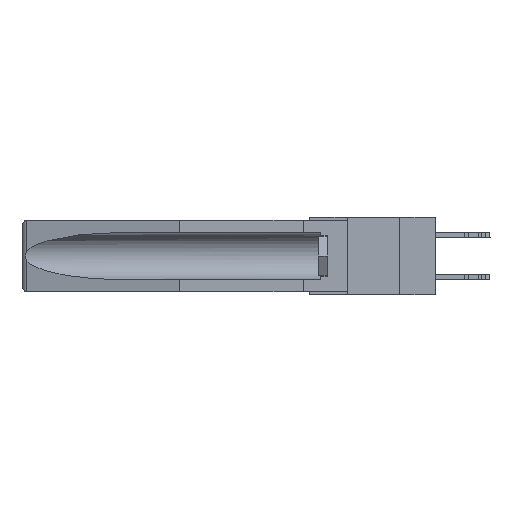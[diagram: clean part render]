
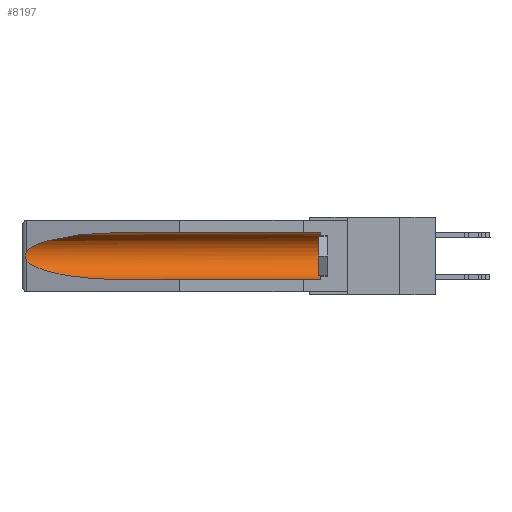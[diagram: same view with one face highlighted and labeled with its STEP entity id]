
A CAD part, left-side view. The second image highlights one B-rep face of the part: STEP entity #8197.
In plain terms, the highlighted cylindrical face has radius 2.857 mm (diameter 5.715 mm), a partial arc.
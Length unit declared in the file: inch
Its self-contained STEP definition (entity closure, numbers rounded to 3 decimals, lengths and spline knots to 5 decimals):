
#488 = CARTESIAN_POINT ( 'NONE',  ( 0.21114, 1.30732, -0.284 ) ) ;
#608 = CARTESIAN_POINT ( 'NONE',  ( 0.25451, 1.48313, -0.24835 ) ) ;
#1193 = CARTESIAN_POINT ( 'NONE',  ( 0.26537, 1.52718, -0.14972 ) ) ;
#1194 = CARTESIAN_POINT ( 'NONE',  ( 0.26537, 1.52718, -0.19328 ) ) ;
#2556 = DIRECTION ( 'NONE',  ( 0., 1., 0. ) ) ;
#3666 = VERTEX_POINT ( 'NONE', #18218 ) ;
#4886 = FACE_OUTER_BOUND ( 'NONE', #32067, .T. ) ;
#5079 = CARTESIAN_POINT ( 'NONE',  ( 0.26537, 1.52718, -0.14972 ) ) ;
#5500 = LINE ( 'NONE', #27120, #18323 ) ;
#5696 = EDGE_CURVE ( 'NONE', #31423, #12326, #31787, .T. ) ;
#6207 = ORIENTED_EDGE ( 'NONE', *, *, #6309, .F. ) ;
#6309 = EDGE_CURVE ( 'NONE', #16053, #23123, #12620, .T. ) ;
#6345 = ORIENTED_EDGE ( 'NONE', *, *, #5696, .T. ) ;
#7160 = CARTESIAN_POINT ( 'NONE',  ( 0.2673, 1.5327, -0.16383 ) ) ;
#7705 = CARTESIAN_POINT ( 'NONE',  ( 0.155, 1.07973, -0.284 ) ) ;
#8197 = ADVANCED_FACE ( 'NONE', ( #4886 ), #17711, .F. ) ;
#8872 = ORIENTED_EDGE ( 'NONE', *, *, #15771, .T. ) ;
#9637 = CARTESIAN_POINT ( 'NONE',  ( 0.26654, 1.53092, -0.15636 ) ) ;
#9998 = DIRECTION ( 'NONE',  ( 0., 0., 1. ) ) ;
#10888 =( BOUNDED_CURVE ( )  B_SPLINE_CURVE ( 3, ( #10934, #608, #488, #23588 ),
 .UNSPECIFIED., .F., .F. ) 
 B_SPLINE_CURVE_WITH_KNOTS ( ( 4, 4 ),
 ( 0.1948, 1.5708 ),
 .UNSPECIFIED. ) 
 CURVE ( )  GEOMETRIC_REPRESENTATION_ITEM ( )  RATIONAL_B_SPLINE_CURVE ( ( 1., 0.848, 0.848, 1. ) ) 
 REPRESENTATION_ITEM ( '' )  );
#10934 = CARTESIAN_POINT ( 'NONE',  ( 0.26537, 1.52718, -0.19328 ) ) ;
#11976 = EDGE_CURVE ( 'NONE', #16053, #21018, #19033, .T. ) ;
#12223 = CARTESIAN_POINT ( 'NONE',  ( 0.155, -0.30754, -0.284 ) ) ;
#12326 = VERTEX_POINT ( 'NONE', #1193 ) ;
#12581 = ORIENTED_EDGE ( 'NONE', *, *, #17469, .T. ) ;
#12620 = LINE ( 'NONE', #12223, #29821 ) ;
#13953 = CARTESIAN_POINT ( 'NONE',  ( 0.26655, 1.53094, -0.18657 ) ) ;
#14879 = CARTESIAN_POINT ( 'NONE',  ( 0.155, 1.07973, -0.059 ) ) ;
#15127 = ORIENTED_EDGE ( 'NONE', *, *, #11976, .T. ) ;
#15260 = DIRECTION ( 'NONE',  ( 0., 1., 0. ) ) ;
#15278 = CARTESIAN_POINT ( 'NONE',  ( 0.25451, 1.48313, -0.09465 ) ) ;
#15771 = EDGE_CURVE ( 'NONE', #12326, #3666, #16846, .T. ) ;
#16053 = VERTEX_POINT ( 'NONE', #25315 ) ;
#16846 = B_SPLINE_CURVE_WITH_KNOTS ( 'NONE', 3,
 ( #27351, #22171, #9637, #7160, #26981, #29516, #27090, #13953, #32079, #1194 ),
 .UNSPECIFIED., .F., .F.,
 ( 4, 2, 2, 2, 4 ),
 ( 0., 0.00029, 0.00058, 0.00087, 0.00117 ),
 .UNSPECIFIED. ) ;
#17469 = EDGE_CURVE ( 'NONE', #3666, #23123, #10888, .T. ) ;
#17711 = CYLINDRICAL_SURFACE ( 'NONE', #21744, 0.1125 ) ;
#18218 = CARTESIAN_POINT ( 'NONE',  ( 0.26537, 1.52718, -0.19328 ) ) ;
#18323 = VECTOR ( 'NONE', #33009, 39.37008 ) ;
#18968 = EDGE_CURVE ( 'NONE', #21018, #31423, #5500, .T. ) ;
#19033 = CIRCLE ( 'NONE', #23303, 0.1125 ) ;
#19790 = DIRECTION ( 'NONE',  ( 0., -1., 0. ) ) ;
#20298 = CARTESIAN_POINT ( 'NONE',  ( 0.155, 1.07973, -0.059 ) ) ;
#21018 = VERTEX_POINT ( 'NONE', #28309 ) ;
#21744 = AXIS2_PLACEMENT_3D ( 'NONE', #25343, #15260, #9998 ) ;
#22171 = CARTESIAN_POINT ( 'NONE',  ( 0.26597, 1.52961, -0.15275 ) ) ;
#22893 = CARTESIAN_POINT ( 'NONE',  ( 0.21114, 1.30732, -0.059 ) ) ;
#23123 = VERTEX_POINT ( 'NONE', #7705 ) ;
#23303 = AXIS2_PLACEMENT_3D ( 'NONE', #29757, #19790, #27648 ) ;
#23588 = CARTESIAN_POINT ( 'NONE',  ( 0.155, 1.07973, -0.284 ) ) ;
#25315 = CARTESIAN_POINT ( 'NONE',  ( 0.155, 0.126, -0.284 ) ) ;
#25343 = CARTESIAN_POINT ( 'NONE',  ( 0.155, -0.30754, -0.1715 ) ) ;
#26981 = CARTESIAN_POINT ( 'NONE',  ( 0.2675, 1.53308, -0.16763 ) ) ;
#27090 = CARTESIAN_POINT ( 'NONE',  ( 0.2673, 1.53269, -0.17917 ) ) ;
#27120 = CARTESIAN_POINT ( 'NONE',  ( 0.155, -0.30754, -0.059 ) ) ;
#27351 = CARTESIAN_POINT ( 'NONE',  ( 0.26537, 1.52718, -0.14972 ) ) ;
#27648 = DIRECTION ( 'NONE',  ( 0., 0., 1. ) ) ;
#28309 = CARTESIAN_POINT ( 'NONE',  ( 0.155, 0.126, -0.059 ) ) ;
#29516 = CARTESIAN_POINT ( 'NONE',  ( 0.2675, 1.53308, -0.17534 ) ) ;
#29757 = CARTESIAN_POINT ( 'NONE',  ( 0.155, 0.126, -0.1715 ) ) ;
#29821 = VECTOR ( 'NONE', #2556, 39.37008 ) ;
#31398 = ORIENTED_EDGE ( 'NONE', *, *, #18968, .T. ) ;
#31423 = VERTEX_POINT ( 'NONE', #14879 ) ;
#31787 =( BOUNDED_CURVE ( )  B_SPLINE_CURVE ( 3, ( #20298, #22893, #15278, #5079 ),
 .UNSPECIFIED., .F., .T. ) 
 B_SPLINE_CURVE_WITH_KNOTS ( ( 4, 4 ),
 ( 4.71239, 6.08839 ),
 .UNSPECIFIED. ) 
 CURVE ( )  GEOMETRIC_REPRESENTATION_ITEM ( )  RATIONAL_B_SPLINE_CURVE ( ( 1., 0.848, 0.848, 1. ) ) 
 REPRESENTATION_ITEM ( '' )  );
#32067 = EDGE_LOOP ( 'NONE', ( #6345, #8872, #12581, #6207, #15127, #31398 ) ) ;
#32079 = CARTESIAN_POINT ( 'NONE',  ( 0.26597, 1.5296, -0.19026 ) ) ;
#33009 = DIRECTION ( 'NONE',  ( 0., 1., 0. ) ) ;
